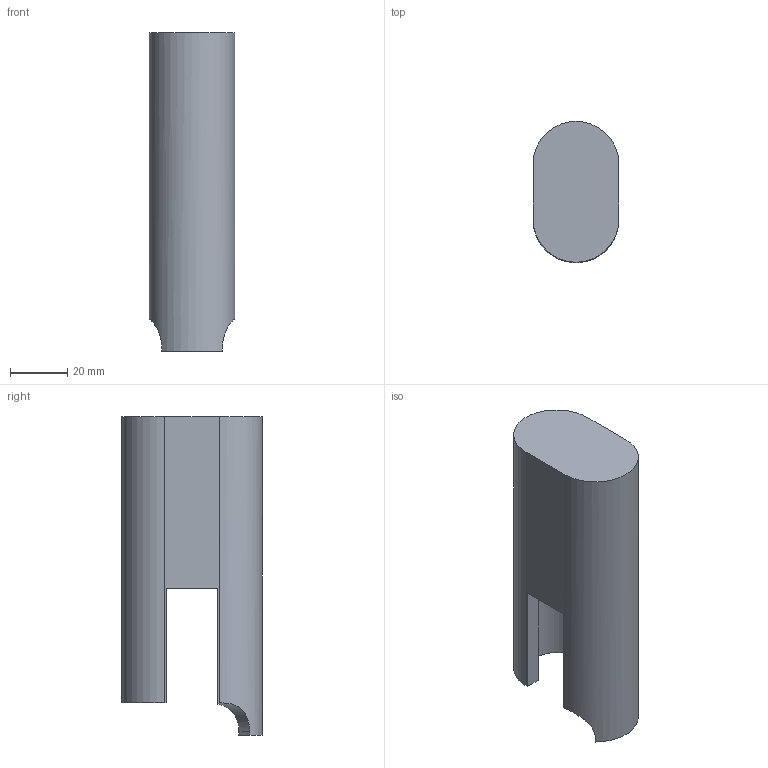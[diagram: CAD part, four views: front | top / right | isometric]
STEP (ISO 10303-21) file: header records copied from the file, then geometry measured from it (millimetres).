
FILE_DESCRIPTION (( 'STEP AP203' ), '1' );
FILE_NAME ('WeldingJig.STEP', '2020-05-19T19:50:58', ( '' ), ( '' ), 'SwSTEP 2.0', 'SolidWorks 2019', '' );
FILE_SCHEMA (( 'CONFIG_CONTROL_DESIGN' ));
Length unit declared in the file: millimetre
Products named in the file (1): WeldingJig
Bounding box: 30 x 49.2 x 111.3 mm (x, y, z)
Volume: 82722.2 mm3; surface area: 21184.4 mm2
Topology: 1 solids, 1 shells, 31 faces, 84 edges, 56 vertices
Faces by surface type: plane 20, cylinder 11
Entity records: 1149 total; most frequent: CARTESIAN_POINT 282, ORIENTED_EDGE 168, DIRECTION 162, EDGE_CURVE 84, VERTEX_POINT 56, LINE 54, AXIS2_PLACEMENT_3D 54, VECTOR 54
